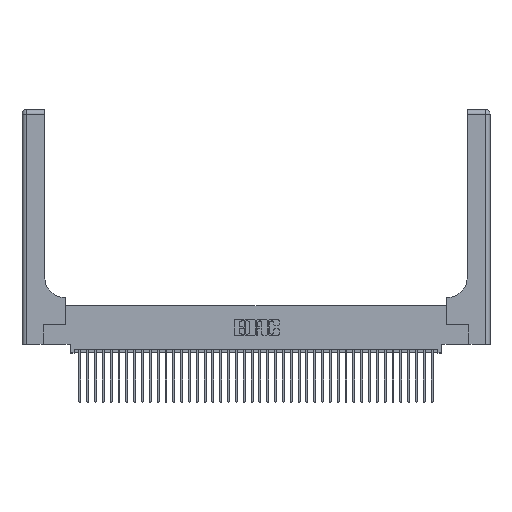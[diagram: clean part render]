
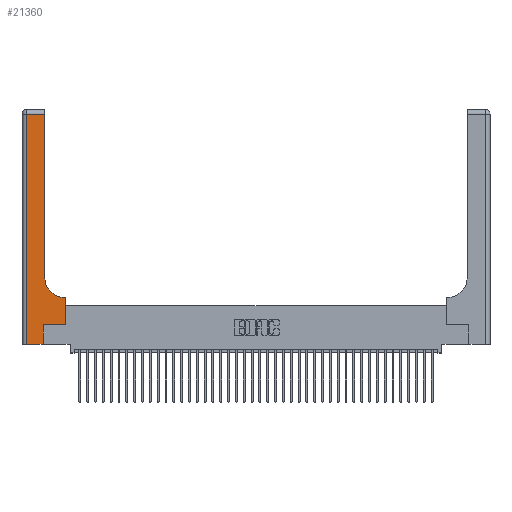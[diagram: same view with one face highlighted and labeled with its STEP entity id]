
A CAD part, top view. The second image highlights one B-rep face of the part: STEP entity #21360.
In plain terms, the highlighted planar face has unit normal (0, 0, 1).
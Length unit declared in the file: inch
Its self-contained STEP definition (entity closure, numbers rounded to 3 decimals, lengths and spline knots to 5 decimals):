
#232 = VECTOR ( 'NONE', #37309, 39.37008 ) ;
#1230 = CARTESIAN_POINT ( 'NONE',  ( 0.5585, 0.25, 0.37 ) ) ;
#1634 = CARTESIAN_POINT ( 'NONE',  ( 0.2915, 0.6, 0.37 ) ) ;
#2181 = CARTESIAN_POINT ( 'NONE',  ( 0.06, 0., 0.37 ) ) ;
#2409 = DIRECTION ( 'NONE',  ( -1., 0., 0. ) ) ;
#2774 = VECTOR ( 'NONE', #7869, 39.37008 ) ;
#3615 = LINE ( 'NONE', #10425, #4615 ) ;
#4154 = CIRCLE ( 'NONE', #17828, 0.25 ) ;
#4432 = DIRECTION ( 'NONE',  ( 0., 1., 0. ) ) ;
#4615 = VECTOR ( 'NONE', #16850, 39.37008 ) ;
#4648 = EDGE_CURVE ( 'NONE', #38764, #26122, #28125, .T. ) ;
#4693 = CARTESIAN_POINT ( 'NONE',  ( 0.269, 0., 0.37 ) ) ;
#4808 = DIRECTION ( 'NONE',  ( -1., 0., 0. ) ) ;
#5198 = LINE ( 'NONE', #1230, #21146 ) ;
#6440 = EDGE_CURVE ( 'NONE', #36012, #23920, #3615, .T. ) ;
#6703 = CARTESIAN_POINT ( 'NONE',  ( 0., 2.94, 0.37 ) ) ;
#7869 = DIRECTION ( 'NONE',  ( 0., 1., 0. ) ) ;
#7944 = CARTESIAN_POINT ( 'NONE',  ( 0.5585, 0.6, 0.37 ) ) ;
#8652 = CARTESIAN_POINT ( 'NONE',  ( 0., 3., 0.37 ) ) ;
#9209 = ORIENTED_EDGE ( 'NONE', *, *, #33051, .T. ) ;
#9919 = DIRECTION ( 'NONE',  ( -1., 0., 0. ) ) ;
#10425 = CARTESIAN_POINT ( 'NONE',  ( 0.06, 3., 0.37 ) ) ;
#11089 = VECTOR ( 'NONE', #31907, 39.37008 ) ;
#11184 = FACE_OUTER_BOUND ( 'NONE', #16484, .T. ) ;
#11279 = CARTESIAN_POINT ( 'NONE',  ( 0.2915, 3., 0.37 ) ) ;
#11415 = EDGE_CURVE ( 'NONE', #21276, #15802, #14357, .T. ) ;
#11474 = CARTESIAN_POINT ( 'NONE',  ( 0.2915, 0.85, 0.37 ) ) ;
#12345 = VERTEX_POINT ( 'NONE', #29313 ) ;
#13357 = VECTOR ( 'NONE', #14486, 39.37008 ) ;
#13762 = CARTESIAN_POINT ( 'NONE',  ( 0.5415, 0.85, 0.37 ) ) ;
#13890 = VERTEX_POINT ( 'NONE', #7944 ) ;
#14357 = LINE ( 'NONE', #11279, #13357 ) ;
#14486 = DIRECTION ( 'NONE',  ( 0., 1., 0. ) ) ;
#15111 = PLANE ( 'NONE',  #30220 ) ;
#15558 = VERTEX_POINT ( 'NONE', #39103 ) ;
#15802 = VERTEX_POINT ( 'NONE', #17229 ) ;
#16089 = ORIENTED_EDGE ( 'NONE', *, *, #6440, .T. ) ;
#16484 = EDGE_LOOP ( 'NONE', ( #17275, #35743, #16089, #9209, #19936, #18433, #30358, #27131, #30955 ) ) ;
#16850 = DIRECTION ( 'NONE',  ( 0., -1., 0. ) ) ;
#16975 = DIRECTION ( 'NONE',  ( 1., 0., 0. ) ) ;
#17229 = CARTESIAN_POINT ( 'NONE',  ( 0.2915, 2.94, 0.37 ) ) ;
#17275 = ORIENTED_EDGE ( 'NONE', *, *, #11415, .T. ) ;
#17828 = AXIS2_PLACEMENT_3D ( 'NONE', #13762, #35758, #16975 ) ;
#18433 = ORIENTED_EDGE ( 'NONE', *, *, #31107, .T. ) ;
#19936 = ORIENTED_EDGE ( 'NONE', *, *, #4648, .T. ) ;
#21146 = VECTOR ( 'NONE', #4432, 39.37008 ) ;
#21276 = VERTEX_POINT ( 'NONE', #11474 ) ;
#21360 = ADVANCED_FACE ( 'NONE', ( #11184 ), #15111, .F. ) ;
#21468 = DIRECTION ( 'NONE',  ( 0., 0., -1. ) ) ;
#21737 = CARTESIAN_POINT ( 'NONE',  ( 0.269, 0.25, 0.37 ) ) ;
#22350 = CARTESIAN_POINT ( 'NONE',  ( 0.269, 0.25, 0.37 ) ) ;
#23571 = LINE ( 'NONE', #1634, #39176 ) ;
#23920 = VERTEX_POINT ( 'NONE', #2181 ) ;
#24221 = VECTOR ( 'NONE', #9919, 39.37008 ) ;
#25222 = LINE ( 'NONE', #6703, #24221 ) ;
#25746 = CARTESIAN_POINT ( 'NONE',  ( 0., 0., 0.37 ) ) ;
#26122 = VERTEX_POINT ( 'NONE', #22350 ) ;
#27131 = ORIENTED_EDGE ( 'NONE', *, *, #32099, .T. ) ;
#28125 = LINE ( 'NONE', #4693, #2774 ) ;
#29313 = CARTESIAN_POINT ( 'NONE',  ( 0.5415, 0.6, 0.37 ) ) ;
#29888 = CARTESIAN_POINT ( 'NONE',  ( 0.269, 0., 0.37 ) ) ;
#29983 = EDGE_CURVE ( 'NONE', #15802, #36012, #25222, .T. ) ;
#30220 = AXIS2_PLACEMENT_3D ( 'NONE', #8652, #21468, #2409 ) ;
#30358 = ORIENTED_EDGE ( 'NONE', *, *, #38068, .T. ) ;
#30955 = ORIENTED_EDGE ( 'NONE', *, *, #31973, .T. ) ;
#31107 = EDGE_CURVE ( 'NONE', #26122, #15558, #33923, .T. ) ;
#31907 = DIRECTION ( 'NONE',  ( 1., 0., 0. ) ) ;
#31973 = EDGE_CURVE ( 'NONE', #12345, #21276, #4154, .T. ) ;
#32099 = EDGE_CURVE ( 'NONE', #13890, #12345, #23571, .T. ) ;
#32762 = CARTESIAN_POINT ( 'NONE',  ( 0.06, 2.94, 0.37 ) ) ;
#33051 = EDGE_CURVE ( 'NONE', #23920, #38764, #34277, .T. ) ;
#33923 = LINE ( 'NONE', #21737, #232 ) ;
#34277 = LINE ( 'NONE', #25746, #11089 ) ;
#35743 = ORIENTED_EDGE ( 'NONE', *, *, #29983, .T. ) ;
#35758 = DIRECTION ( 'NONE',  ( 0., 0., -1. ) ) ;
#36012 = VERTEX_POINT ( 'NONE', #32762 ) ;
#37309 = DIRECTION ( 'NONE',  ( 1., 0., 0. ) ) ;
#38068 = EDGE_CURVE ( 'NONE', #15558, #13890, #5198, .T. ) ;
#38764 = VERTEX_POINT ( 'NONE', #29888 ) ;
#39103 = CARTESIAN_POINT ( 'NONE',  ( 0.5585, 0.25, 0.37 ) ) ;
#39176 = VECTOR ( 'NONE', #4808, 39.37008 ) ;
